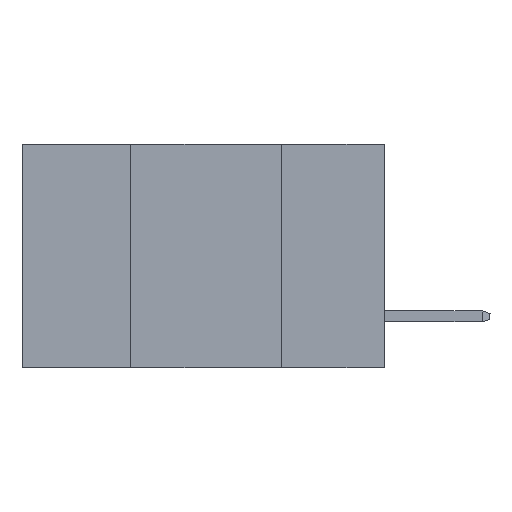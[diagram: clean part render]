
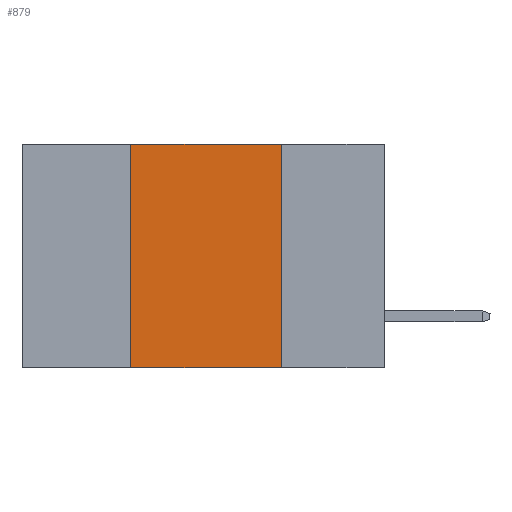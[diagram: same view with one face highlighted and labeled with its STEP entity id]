
A CAD part, left-side view. The second image highlights one B-rep face of the part: STEP entity #879.
In plain terms, the highlighted planar face has unit normal (-1, 0, 0).
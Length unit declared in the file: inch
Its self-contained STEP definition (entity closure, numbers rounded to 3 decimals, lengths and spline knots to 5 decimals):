
#58 = ORIENTED_EDGE ( 'NONE', *, *, #18945, .F. ) ;
#879 = ADVANCED_FACE ( 'NONE', ( #19826 ), #10449, .F. ) ;
#1025 = CARTESIAN_POINT ( 'NONE',  ( 0., 0.6, 0. ) ) ;
#1028 = DIRECTION ( 'NONE',  ( 0., -1., 0. ) ) ;
#1933 = VERTEX_POINT ( 'NONE', #7860 ) ;
#2077 = EDGE_CURVE ( 'NONE', #1933, #3635, #15893, .T. ) ;
#2613 = VERTEX_POINT ( 'NONE', #8081 ) ;
#2693 = CARTESIAN_POINT ( 'NONE',  ( 0., 0.17, -0.37 ) ) ;
#3635 = VERTEX_POINT ( 'NONE', #6119 ) ;
#4769 = VECTOR ( 'NONE', #6228, 39.37008 ) ;
#6119 = CARTESIAN_POINT ( 'NONE',  ( 0., 0.17, 0. ) ) ;
#6228 = DIRECTION ( 'NONE',  ( 0., -1., 0. ) ) ;
#7860 = CARTESIAN_POINT ( 'NONE',  ( 0., 0.42, 0. ) ) ;
#8081 = CARTESIAN_POINT ( 'NONE',  ( 0., 0.42, -0.37 ) ) ;
#8205 = VERTEX_POINT ( 'NONE', #17434 ) ;
#8602 = DIRECTION ( 'NONE',  ( 1., 0., 0. ) ) ;
#8799 = ORIENTED_EDGE ( 'NONE', *, *, #22036, .T. ) ;
#9329 = VECTOR ( 'NONE', #21325, 39.37008 ) ;
#10253 = LINE ( 'NONE', #2693, #18291 ) ;
#10449 = PLANE ( 'NONE',  #12724 ) ;
#10868 = ORIENTED_EDGE ( 'NONE', *, *, #14904, .F. ) ;
#11649 = ORIENTED_EDGE ( 'NONE', *, *, #2077, .F. ) ;
#12555 = EDGE_LOOP ( 'NONE', ( #10868, #11649, #58, #8799 ) ) ;
#12724 = AXIS2_PLACEMENT_3D ( 'NONE', #1025, #8602, #16137 ) ;
#14904 = EDGE_CURVE ( 'NONE', #3635, #8205, #10253, .T. ) ;
#15658 = LINE ( 'NONE', #23189, #4769 ) ;
#15893 = LINE ( 'NONE', #17632, #24137 ) ;
#16137 = DIRECTION ( 'NONE',  ( 0., 0., -1. ) ) ;
#17278 = LINE ( 'NONE', #20959, #9329 ) ;
#17434 = CARTESIAN_POINT ( 'NONE',  ( 0., 0.17, -0.37 ) ) ;
#17632 = CARTESIAN_POINT ( 'NONE',  ( 0., 0.6, 0. ) ) ;
#17796 = DIRECTION ( 'NONE',  ( 0., 0., -1. ) ) ;
#18291 = VECTOR ( 'NONE', #17796, 39.37008 ) ;
#18945 = EDGE_CURVE ( 'NONE', #2613, #1933, #17278, .T. ) ;
#19826 = FACE_OUTER_BOUND ( 'NONE', #12555, .T. ) ;
#20959 = CARTESIAN_POINT ( 'NONE',  ( 0., 0.42, -0.37 ) ) ;
#21325 = DIRECTION ( 'NONE',  ( 0., 0., 1. ) ) ;
#22036 = EDGE_CURVE ( 'NONE', #2613, #8205, #15658, .T. ) ;
#23189 = CARTESIAN_POINT ( 'NONE',  ( 0., 0.6, -0.37 ) ) ;
#24137 = VECTOR ( 'NONE', #1028, 39.37008 ) ;
